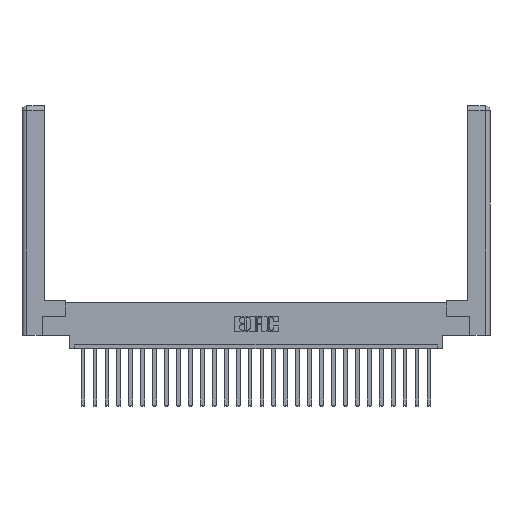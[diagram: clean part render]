
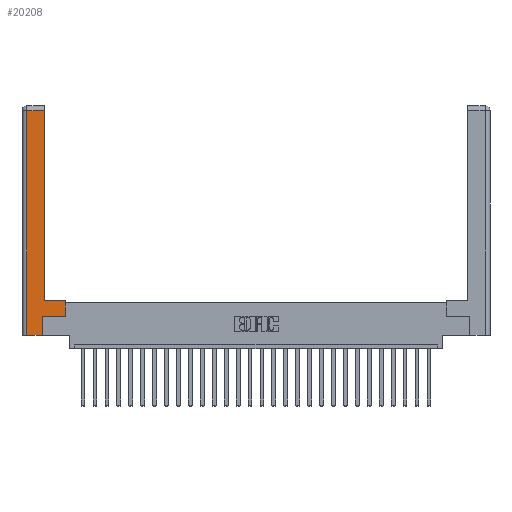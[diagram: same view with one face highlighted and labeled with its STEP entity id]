
A CAD part, top view. The second image highlights one B-rep face of the part: STEP entity #20208.
In plain terms, the highlighted planar face has unit normal (0, 0, 1).
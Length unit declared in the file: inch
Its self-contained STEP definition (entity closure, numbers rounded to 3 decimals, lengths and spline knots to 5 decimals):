
#144 = DIRECTION ( 'NONE',  ( -1., 0., 0. ) ) ;
#365 = CARTESIAN_POINT ( 'NONE',  ( 0.0615, 0., 0. ) ) ;
#379 = VERTEX_POINT ( 'NONE', #7953 ) ;
#1202 = DIRECTION ( 'NONE',  ( 0., -1., 0. ) ) ;
#1510 = CARTESIAN_POINT ( 'NONE',  ( 0.565, 0.245, 0. ) ) ;
#1703 = CARTESIAN_POINT ( 'NONE',  ( 0.0615, 2.94, 0. ) ) ;
#2288 = LINE ( 'NONE', #1703, #17926 ) ;
#2454 = VECTOR ( 'NONE', #1202, 39.37008 ) ;
#4387 = ORIENTED_EDGE ( 'NONE', *, *, #25471, .T. ) ;
#4422 = DIRECTION ( 'NONE',  ( 0., 1., 0. ) ) ;
#4634 = CARTESIAN_POINT ( 'NONE',  ( 0.295, 0.45, 0. ) ) ;
#4793 = LINE ( 'NONE', #10286, #15584 ) ;
#4811 = VECTOR ( 'NONE', #18776, 39.37008 ) ;
#4828 = ORIENTED_EDGE ( 'NONE', *, *, #17601, .T. ) ;
#4830 = LINE ( 'NONE', #16162, #15939 ) ;
#5388 = EDGE_CURVE ( 'NONE', #25013, #7293, #11809, .T. ) ;
#5457 = CARTESIAN_POINT ( 'NONE',  ( 0.0615, 0., 0. ) ) ;
#5505 = EDGE_CURVE ( 'NONE', #23098, #9343, #4830, .T. ) ;
#6317 = EDGE_CURVE ( 'NONE', #16925, #11444, #14003, .T. ) ;
#6937 = LINE ( 'NONE', #4634, #9767 ) ;
#7293 = VERTEX_POINT ( 'NONE', #9886 ) ;
#7296 = CARTESIAN_POINT ( 'NONE',  ( 0.265, 0., 0. ) ) ;
#7875 = EDGE_CURVE ( 'NONE', #7293, #379, #2288, .T. ) ;
#7953 = CARTESIAN_POINT ( 'NONE',  ( 0.0615, 2.94, 0. ) ) ;
#8204 = ORIENTED_EDGE ( 'NONE', *, *, #5388, .T. ) ;
#8720 = DIRECTION ( 'NONE',  ( -1., 0., 0. ) ) ;
#8874 = EDGE_CURVE ( 'NONE', #11444, #13537, #4793, .T. ) ;
#9265 = AXIS2_PLACEMENT_3D ( 'NONE', #14363, #12596, #144 ) ;
#9343 = VERTEX_POINT ( 'NONE', #23969 ) ;
#9731 = CARTESIAN_POINT ( 'NONE',  ( 0.295, 3., 0. ) ) ;
#9767 = VECTOR ( 'NONE', #8720, 39.37008 ) ;
#9886 = CARTESIAN_POINT ( 'NONE',  ( 0.295, 2.94, 0. ) ) ;
#10286 = CARTESIAN_POINT ( 'NONE',  ( 0.265, 0.245, 0. ) ) ;
#10619 = EDGE_LOOP ( 'NONE', ( #8204, #26377, #4828, #25139, #23131, #22965, #20163, #4387 ) ) ;
#10780 = CARTESIAN_POINT ( 'NONE',  ( 0.265, 0., 0. ) ) ;
#11444 = VERTEX_POINT ( 'NONE', #7296 ) ;
#11809 = LINE ( 'NONE', #9731, #19539 ) ;
#12062 = FACE_OUTER_BOUND ( 'NONE', #10619, .T. ) ;
#12596 = DIRECTION ( 'NONE',  ( 0., 0., -1. ) ) ;
#13537 = VERTEX_POINT ( 'NONE', #25240 ) ;
#14003 = LINE ( 'NONE', #10780, #4811 ) ;
#14363 = CARTESIAN_POINT ( 'NONE',  ( 0., 0., 0. ) ) ;
#15584 = VECTOR ( 'NONE', #4422, 39.37008 ) ;
#15703 = DIRECTION ( 'NONE',  ( 0., 1., 0. ) ) ;
#15939 = VECTOR ( 'NONE', #18517, 39.37008 ) ;
#16162 = CARTESIAN_POINT ( 'NONE',  ( 0.565, 0.45, 0. ) ) ;
#16925 = VERTEX_POINT ( 'NONE', #365 ) ;
#17601 = EDGE_CURVE ( 'NONE', #379, #16925, #20336, .T. ) ;
#17926 = VECTOR ( 'NONE', #20287, 39.37008 ) ;
#18376 = EDGE_CURVE ( 'NONE', #13537, #23098, #19045, .T. ) ;
#18452 = DIRECTION ( 'NONE',  ( 1., 0., 0. ) ) ;
#18517 = DIRECTION ( 'NONE',  ( 0., 1., 0. ) ) ;
#18636 = CARTESIAN_POINT ( 'NONE',  ( 0.565, 0.245, 0. ) ) ;
#18776 = DIRECTION ( 'NONE',  ( 1., 0., 0. ) ) ;
#18804 = PLANE ( 'NONE',  #9265 ) ;
#19045 = LINE ( 'NONE', #18636, #26013 ) ;
#19539 = VECTOR ( 'NONE', #15703, 39.37008 ) ;
#20163 = ORIENTED_EDGE ( 'NONE', *, *, #5505, .T. ) ;
#20208 = ADVANCED_FACE ( 'NONE', ( #12062 ), #18804, .F. ) ;
#20287 = DIRECTION ( 'NONE',  ( -1., 0., 0. ) ) ;
#20336 = LINE ( 'NONE', #5457, #2454 ) ;
#22965 = ORIENTED_EDGE ( 'NONE', *, *, #18376, .T. ) ;
#23098 = VERTEX_POINT ( 'NONE', #1510 ) ;
#23131 = ORIENTED_EDGE ( 'NONE', *, *, #8874, .T. ) ;
#23969 = CARTESIAN_POINT ( 'NONE',  ( 0.565, 0.45, 0. ) ) ;
#25013 = VERTEX_POINT ( 'NONE', #26050 ) ;
#25139 = ORIENTED_EDGE ( 'NONE', *, *, #6317, .T. ) ;
#25240 = CARTESIAN_POINT ( 'NONE',  ( 0.265, 0.245, 0. ) ) ;
#25471 = EDGE_CURVE ( 'NONE', #9343, #25013, #6937, .T. ) ;
#26013 = VECTOR ( 'NONE', #18452, 39.37008 ) ;
#26050 = CARTESIAN_POINT ( 'NONE',  ( 0.295, 0.45, 0. ) ) ;
#26377 = ORIENTED_EDGE ( 'NONE', *, *, #7875, .T. ) ;
